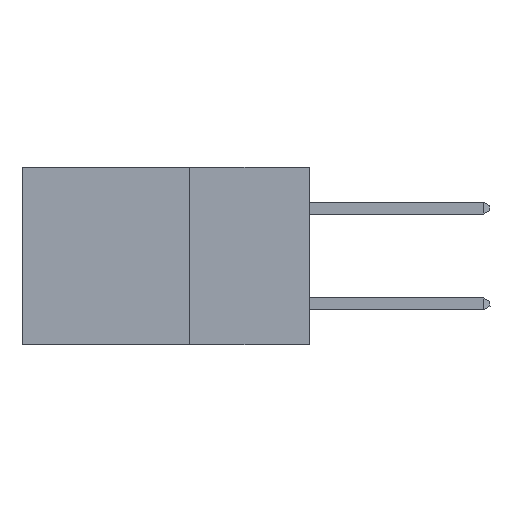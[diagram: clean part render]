
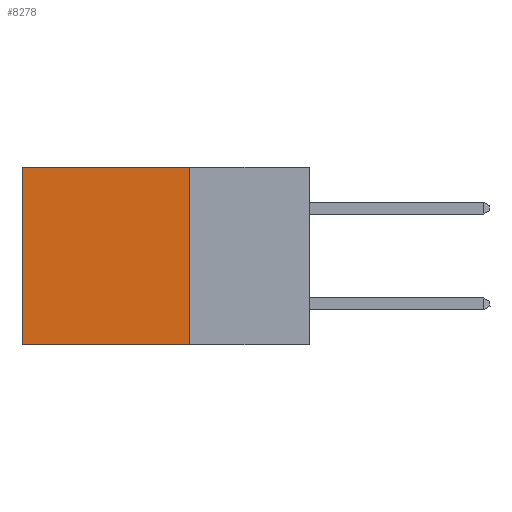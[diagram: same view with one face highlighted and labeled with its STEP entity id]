
A CAD part, left-side view. The second image highlights one B-rep face of the part: STEP entity #8278.
In plain terms, the highlighted planar face has unit normal (-1, 0, 0).
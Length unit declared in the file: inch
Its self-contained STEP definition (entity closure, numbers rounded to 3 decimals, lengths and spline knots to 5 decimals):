
#357 = EDGE_CURVE ( 'NONE', #8896, #11414, #15437, .T. ) ;
#806 = CARTESIAN_POINT ( 'NONE',  ( 0.2875, 0.25, 0. ) ) ;
#879 = CARTESIAN_POINT ( 'NONE',  ( 0.2875, 0.25, -0.37 ) ) ;
#1276 = CARTESIAN_POINT ( 'NONE',  ( 0.2875, 0.25, 0. ) ) ;
#1602 = EDGE_CURVE ( 'NONE', #7397, #11414, #15398, .T. ) ;
#1805 = VERTEX_POINT ( 'NONE', #1276 ) ;
#1884 = FACE_OUTER_BOUND ( 'NONE', #13426, .T. ) ;
#2576 = EDGE_CURVE ( 'NONE', #1805, #7397, #3630, .T. ) ;
#3338 = CARTESIAN_POINT ( 'NONE',  ( 0.2875, 0.25, 0. ) ) ;
#3630 = LINE ( 'NONE', #3338, #15177 ) ;
#3754 = ORIENTED_EDGE ( 'NONE', *, *, #357, .F. ) ;
#3950 = LINE ( 'NONE', #12292, #11605 ) ;
#4275 = ORIENTED_EDGE ( 'NONE', *, *, #1602, .T. ) ;
#4365 = CARTESIAN_POINT ( 'NONE',  ( 0.2875, 0.6, -0.37 ) ) ;
#4428 = DIRECTION ( 'NONE',  ( 1., 0., 0. ) ) ;
#4955 = DIRECTION ( 'NONE',  ( 0., 0., -1. ) ) ;
#5106 = EDGE_CURVE ( 'NONE', #1805, #8896, #3950, .T. ) ;
#5747 = VECTOR ( 'NONE', #14024, 39.37008 ) ;
#7397 = VERTEX_POINT ( 'NONE', #9632 ) ;
#8278 = ADVANCED_FACE ( 'NONE', ( #1884 ), #9173, .F. ) ;
#8896 = VERTEX_POINT ( 'NONE', #11834 ) ;
#9173 = PLANE ( 'NONE',  #12404 ) ;
#9632 = CARTESIAN_POINT ( 'NONE',  ( 0.2875, 0.6, 0. ) ) ;
#9634 = CARTESIAN_POINT ( 'NONE',  ( 0.2875, 0.6, 0. ) ) ;
#10062 = ORIENTED_EDGE ( 'NONE', *, *, #2576, .T. ) ;
#10837 = ORIENTED_EDGE ( 'NONE', *, *, #5106, .F. ) ;
#11414 = VERTEX_POINT ( 'NONE', #4365 ) ;
#11605 = VECTOR ( 'NONE', #13447, 39.37008 ) ;
#11834 = CARTESIAN_POINT ( 'NONE',  ( 0.2875, 0.25, -0.37 ) ) ;
#12292 = CARTESIAN_POINT ( 'NONE',  ( 0.2875, 0.25, 0. ) ) ;
#12404 = AXIS2_PLACEMENT_3D ( 'NONE', #806, #4428, #15245 ) ;
#12425 = VECTOR ( 'NONE', #4955, 39.37008 ) ;
#12895 = DIRECTION ( 'NONE',  ( 0., 1., 0. ) ) ;
#13426 = EDGE_LOOP ( 'NONE', ( #4275, #3754, #10837, #10062 ) ) ;
#13447 = DIRECTION ( 'NONE',  ( 0., 0., -1. ) ) ;
#14024 = DIRECTION ( 'NONE',  ( 0., 1., 0. ) ) ;
#15177 = VECTOR ( 'NONE', #12895, 39.37008 ) ;
#15245 = DIRECTION ( 'NONE',  ( 0., 0., -1. ) ) ;
#15398 = LINE ( 'NONE', #9634, #12425 ) ;
#15437 = LINE ( 'NONE', #879, #5747 ) ;
